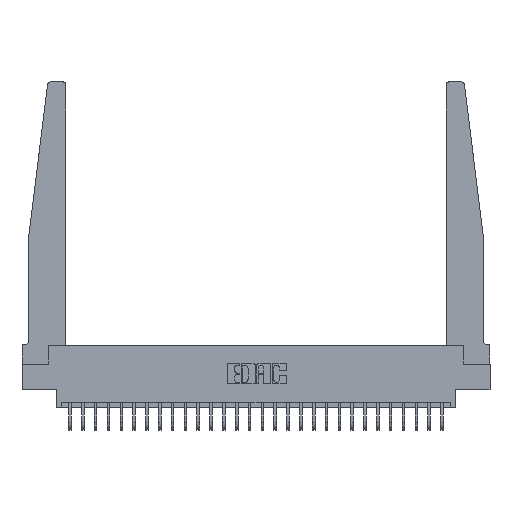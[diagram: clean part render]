
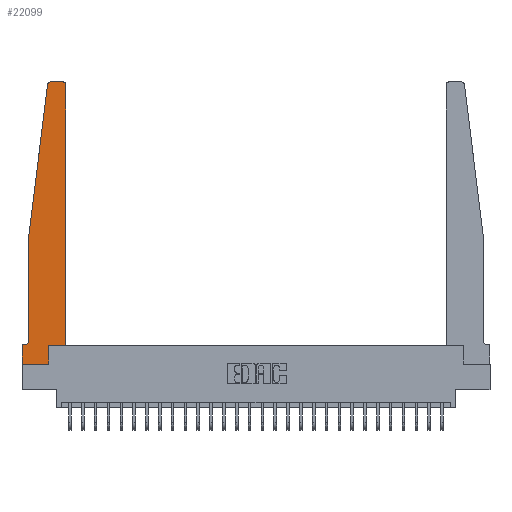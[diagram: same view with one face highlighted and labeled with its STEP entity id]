
A CAD part, top view. The second image highlights one B-rep face of the part: STEP entity #22099.
In plain terms, the highlighted planar face has unit normal (0, 0, 1).
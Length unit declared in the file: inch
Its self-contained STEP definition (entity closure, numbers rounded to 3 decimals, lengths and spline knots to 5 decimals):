
#360 = DIRECTION ( 'NONE',  ( 0., 0., -1. ) ) ;
#669 = VECTOR ( 'NONE', #26770, 39.37008 ) ;
#840 = DIRECTION ( 'NONE',  ( 1., 0., 0. ) ) ;
#971 = LINE ( 'NONE', #7700, #669 ) ;
#1083 = DIRECTION ( 'NONE',  ( -0.122, -0.992, 0. ) ) ;
#1519 = LINE ( 'NONE', #3294, #18076 ) ;
#1800 = ORIENTED_EDGE ( 'NONE', *, *, #4078, .T. ) ;
#2044 = EDGE_CURVE ( 'NONE', #9192, #25907, #11873, .T. ) ;
#2073 = LINE ( 'NONE', #3778, #10804 ) ;
#2210 = EDGE_CURVE ( 'NONE', #7350, #17410, #16284, .T. ) ;
#2533 = VECTOR ( 'NONE', #22319, 39.37008 ) ;
#2592 = LINE ( 'NONE', #16266, #11698 ) ;
#2717 = CARTESIAN_POINT ( 'NONE',  ( 0.065, 0.1875, 0.37 ) ) ;
#3008 = ORIENTED_EDGE ( 'NONE', *, *, #2044, .T. ) ;
#3294 = CARTESIAN_POINT ( 'NONE',  ( 0.25, 2.75, 0.37 ) ) ;
#3310 = EDGE_CURVE ( 'NONE', #7026, #23414, #10441, .T. ) ;
#3778 = CARTESIAN_POINT ( 'NONE',  ( 0., 0., 0.37 ) ) ;
#4078 = EDGE_CURVE ( 'NONE', #11245, #7026, #971, .T. ) ;
#4154 = EDGE_CURVE ( 'NONE', #15787, #9425, #12114, .T. ) ;
#4175 = CARTESIAN_POINT ( 'NONE',  ( 0., 0.1875, 0.37 ) ) ;
#4205 = CARTESIAN_POINT ( 'NONE',  ( 0.425, 0.18, 0.37 ) ) ;
#4708 = AXIS2_PLACEMENT_3D ( 'NONE', #4175, #23732, #25616 ) ;
#4809 = CARTESIAN_POINT ( 'NONE',  ( 0.015, 0.1875, 0.37 ) ) ;
#4830 = CARTESIAN_POINT ( 'NONE',  ( 0.065, 0.2375, 0.37 ) ) ;
#5364 = CARTESIAN_POINT ( 'NONE',  ( 0.27653, 2.72, 0.37 ) ) ;
#5759 = ORIENTED_EDGE ( 'NONE', *, *, #2210, .T. ) ;
#6002 = CARTESIAN_POINT ( 'NONE',  ( 0.395, 2.75, 0.37 ) ) ;
#6030 = EDGE_CURVE ( 'NONE', #7944, #7350, #19149, .T. ) ;
#6044 = CARTESIAN_POINT ( 'NONE',  ( 0., 0.1875, 0.37 ) ) ;
#6112 = EDGE_CURVE ( 'NONE', #23414, #15787, #25840, .T. ) ;
#6314 = ORIENTED_EDGE ( 'NONE', *, *, #4154, .T. ) ;
#6667 = ORIENTED_EDGE ( 'NONE', *, *, #6030, .T. ) ;
#6742 = FACE_OUTER_BOUND ( 'NONE', #24453, .T. ) ;
#6861 = CARTESIAN_POINT ( 'NONE',  ( 0.425, 0.18, 0.37 ) ) ;
#6987 = DIRECTION ( 'NONE',  ( -1., 0., 0. ) ) ;
#7026 = VERTEX_POINT ( 'NONE', #4830 ) ;
#7350 = VERTEX_POINT ( 'NONE', #24690 ) ;
#7521 = CARTESIAN_POINT ( 'NONE',  ( 0., 0., 0.37 ) ) ;
#7700 = CARTESIAN_POINT ( 'NONE',  ( 0.065, 1.25, 0.37 ) ) ;
#7944 = VERTEX_POINT ( 'NONE', #4205 ) ;
#8562 = CARTESIAN_POINT ( 'NONE',  ( 0.395, 2.72, 0.37 ) ) ;
#8714 = EDGE_CURVE ( 'NONE', #9425, #16110, #2073, .T. ) ;
#8938 = CARTESIAN_POINT ( 'NONE',  ( 0.065, 1.25, 0.37 ) ) ;
#9192 = VERTEX_POINT ( 'NONE', #15242 ) ;
#9308 = VECTOR ( 'NONE', #18631, 39.37008 ) ;
#9425 = VERTEX_POINT ( 'NONE', #7521 ) ;
#9605 = CARTESIAN_POINT ( 'NONE',  ( 0.24675, 2.72367, 0.37 ) ) ;
#9972 = CARTESIAN_POINT ( 'NONE',  ( 0.2605, 0., 0.37 ) ) ;
#10224 = EDGE_CURVE ( 'NONE', #16110, #27520, #21500, .T. ) ;
#10441 = CIRCLE ( 'NONE', #13118, 0.05 ) ;
#10639 = CARTESIAN_POINT ( 'NONE',  ( 0.2605, 0.18, 0.37 ) ) ;
#10804 = VECTOR ( 'NONE', #18876, 39.37008 ) ;
#10997 = DIRECTION ( 'NONE',  ( -1., 0., 0. ) ) ;
#11039 = EDGE_CURVE ( 'NONE', #27520, #7944, #18772, .T. ) ;
#11245 = VERTEX_POINT ( 'NONE', #8938 ) ;
#11666 = DIRECTION ( 'NONE',  ( 0., 0., 1. ) ) ;
#11698 = VECTOR ( 'NONE', #1083, 39.37008 ) ;
#11813 = DIRECTION ( 'NONE',  ( 0., -1., 0. ) ) ;
#11873 = CIRCLE ( 'NONE', #24975, 0.03 ) ;
#12114 = LINE ( 'NONE', #13714, #20224 ) ;
#12197 = ORIENTED_EDGE ( 'NONE', *, *, #3310, .T. ) ;
#12920 = PLANE ( 'NONE',  #4708 ) ;
#13118 = AXIS2_PLACEMENT_3D ( 'NONE', #24098, #360, #6987 ) ;
#13379 = VECTOR ( 'NONE', #19366, 39.37008 ) ;
#13714 = CARTESIAN_POINT ( 'NONE',  ( 0., 0., 0.37 ) ) ;
#13843 = ORIENTED_EDGE ( 'NONE', *, *, #8714, .T. ) ;
#13943 = DIRECTION ( 'NONE',  ( -1., 0., 0. ) ) ;
#15242 = CARTESIAN_POINT ( 'NONE',  ( 0.27653, 2.75, 0.37 ) ) ;
#15487 = ORIENTED_EDGE ( 'NONE', *, *, #25901, .T. ) ;
#15787 = VERTEX_POINT ( 'NONE', #6044 ) ;
#16110 = VERTEX_POINT ( 'NONE', #9972 ) ;
#16266 = CARTESIAN_POINT ( 'NONE',  ( 0.065, 1.25, 0.37 ) ) ;
#16284 = CIRCLE ( 'NONE', #19106, 0.03 ) ;
#17410 = VERTEX_POINT ( 'NONE', #6002 ) ;
#18076 = VECTOR ( 'NONE', #13943, 39.37008 ) ;
#18311 = DIRECTION ( 'NONE',  ( 1., 0., 0. ) ) ;
#18631 = DIRECTION ( 'NONE',  ( 0., 1., 0. ) ) ;
#18772 = LINE ( 'NONE', #6861, #2533 ) ;
#18876 = DIRECTION ( 'NONE',  ( 1., 0., 0. ) ) ;
#19106 = AXIS2_PLACEMENT_3D ( 'NONE', #8562, #27297, #18311 ) ;
#19149 = LINE ( 'NONE', #23561, #13379 ) ;
#19366 = DIRECTION ( 'NONE',  ( 0., 1., 0. ) ) ;
#20174 = VECTOR ( 'NONE', #10997, 39.37008 ) ;
#20224 = VECTOR ( 'NONE', #11813, 39.37008 ) ;
#21500 = LINE ( 'NONE', #22323, #9308 ) ;
#22099 = ADVANCED_FACE ( 'NONE', ( #6742 ), #12920, .T. ) ;
#22319 = DIRECTION ( 'NONE',  ( 1., 0., 0. ) ) ;
#22323 = CARTESIAN_POINT ( 'NONE',  ( 0.2605, 0.18, 0.37 ) ) ;
#23414 = VERTEX_POINT ( 'NONE', #4809 ) ;
#23539 = ORIENTED_EDGE ( 'NONE', *, *, #10224, .T. ) ;
#23561 = CARTESIAN_POINT ( 'NONE',  ( 0.425, 0.18, 0.37 ) ) ;
#23732 = DIRECTION ( 'NONE',  ( 0., 0., 1. ) ) ;
#23822 = ORIENTED_EDGE ( 'NONE', *, *, #11039, .T. ) ;
#24098 = CARTESIAN_POINT ( 'NONE',  ( 0.015, 0.2375, 0.37 ) ) ;
#24232 = EDGE_CURVE ( 'NONE', #25907, #11245, #2592, .T. ) ;
#24423 = ORIENTED_EDGE ( 'NONE', *, *, #24232, .T. ) ;
#24453 = EDGE_LOOP ( 'NONE', ( #15487, #3008, #24423, #1800, #12197, #26666, #6314, #13843, #23539, #23822, #6667, #5759 ) ) ;
#24690 = CARTESIAN_POINT ( 'NONE',  ( 0.425, 2.72, 0.37 ) ) ;
#24975 = AXIS2_PLACEMENT_3D ( 'NONE', #5364, #11666, #840 ) ;
#25616 = DIRECTION ( 'NONE',  ( 1., 0., 0. ) ) ;
#25840 = LINE ( 'NONE', #2717, #20174 ) ;
#25901 = EDGE_CURVE ( 'NONE', #17410, #9192, #1519, .T. ) ;
#25907 = VERTEX_POINT ( 'NONE', #9605 ) ;
#26666 = ORIENTED_EDGE ( 'NONE', *, *, #6112, .T. ) ;
#26770 = DIRECTION ( 'NONE',  ( 0., -1., 0. ) ) ;
#27297 = DIRECTION ( 'NONE',  ( 0., 0., 1. ) ) ;
#27520 = VERTEX_POINT ( 'NONE', #10639 ) ;
